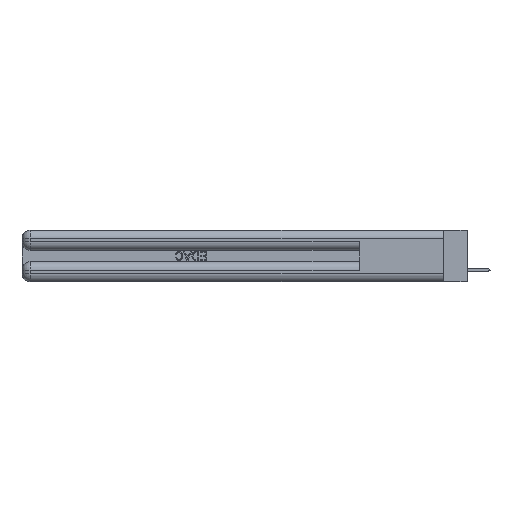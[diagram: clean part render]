
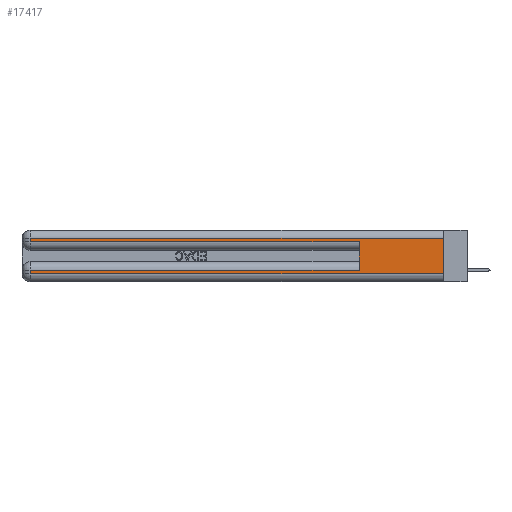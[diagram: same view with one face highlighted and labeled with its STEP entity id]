
A CAD part, left-side view. The second image highlights one B-rep face of the part: STEP entity #17417.
In plain terms, the highlighted planar face has unit normal (-1, 0, 0).
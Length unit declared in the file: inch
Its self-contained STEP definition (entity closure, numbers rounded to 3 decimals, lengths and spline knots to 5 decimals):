
#682 = VERTEX_POINT ( 'NONE', #5060 ) ;
#722 = DIRECTION ( 'NONE',  ( 0., -1., 0. ) ) ;
#943 = ORIENTED_EDGE ( 'NONE', *, *, #21924, .T. ) ;
#945 = DIRECTION ( 'NONE',  ( 0., 0., -1. ) ) ;
#1833 = DIRECTION ( 'NONE',  ( 0., 1., 0. ) ) ;
#3989 = ORIENTED_EDGE ( 'NONE', *, *, #22586, .T. ) ;
#4301 = DIRECTION ( 'NONE',  ( 0., 0., -1. ) ) ;
#4727 = CARTESIAN_POINT ( 'NONE',  ( 0., 0., 0.085 ) ) ;
#5060 = CARTESIAN_POINT ( 'NONE',  ( 0., 0.6, 0.085 ) ) ;
#5175 = CARTESIAN_POINT ( 'NONE',  ( 0., 2.94, 0.31 ) ) ;
#5986 = EDGE_LOOP ( 'NONE', ( #32829, #24049, #3989, #37953, #37852, #943, #38715, #15511 ) ) ;
#6036 = DIRECTION ( 'NONE',  ( 0., -1., 0. ) ) ;
#8787 = DIRECTION ( 'NONE',  ( 0., 0., 1. ) ) ;
#9273 = EDGE_CURVE ( 'NONE', #23100, #13949, #23487, .T. ) ;
#9518 = VERTEX_POINT ( 'NONE', #26101 ) ;
#10511 = EDGE_CURVE ( 'NONE', #9518, #33325, #34875, .T. ) ;
#10585 = DIRECTION ( 'NONE',  ( 1., 0., 0. ) ) ;
#11174 = EDGE_CURVE ( 'NONE', #23100, #39749, #25785, .T. ) ;
#11259 = CARTESIAN_POINT ( 'NONE',  ( 0., 0., 0.06 ) ) ;
#13336 = CARTESIAN_POINT ( 'NONE',  ( 0., 2.94, 0.37 ) ) ;
#13949 = VERTEX_POINT ( 'NONE', #11259 ) ;
#13953 = PLANE ( 'NONE',  #19264 ) ;
#14038 = DIRECTION ( 'NONE',  ( 0., 0., -1. ) ) ;
#14986 = VECTOR ( 'NONE', #8787, 39.37008 ) ;
#15511 = ORIENTED_EDGE ( 'NONE', *, *, #22435, .T. ) ;
#17315 = DIRECTION ( 'NONE',  ( 0., 0., -1. ) ) ;
#17417 = ADVANCED_FACE ( 'NONE', ( #29354 ), #13953, .F. ) ;
#17633 = CARTESIAN_POINT ( 'NONE',  ( 0., 2.94, 0.06 ) ) ;
#18669 = LINE ( 'NONE', #19816, #22580 ) ;
#19074 = VECTOR ( 'NONE', #14038, 39.37008 ) ;
#19264 = AXIS2_PLACEMENT_3D ( 'NONE', #36250, #10585, #17315 ) ;
#19464 = LINE ( 'NONE', #41075, #25459 ) ;
#19816 = CARTESIAN_POINT ( 'NONE',  ( 0., 0., 0.06 ) ) ;
#21317 = CARTESIAN_POINT ( 'NONE',  ( 0., 0.6, 0.145 ) ) ;
#21924 = EDGE_CURVE ( 'NONE', #682, #9518, #28683, .T. ) ;
#22400 = LINE ( 'NONE', #21317, #14986 ) ;
#22435 = EDGE_CURVE ( 'NONE', #33325, #13949, #18669, .T. ) ;
#22580 = VECTOR ( 'NONE', #722, 39.37008 ) ;
#22586 = EDGE_CURVE ( 'NONE', #39749, #40207, #29570, .T. ) ;
#23100 = VERTEX_POINT ( 'NONE', #27547 ) ;
#23487 = LINE ( 'NONE', #33095, #19074 ) ;
#23728 = CARTESIAN_POINT ( 'NONE',  ( 0., 2.94, 0.285 ) ) ;
#24049 = ORIENTED_EDGE ( 'NONE', *, *, #11174, .T. ) ;
#25459 = VECTOR ( 'NONE', #6036, 39.37008 ) ;
#25625 = VECTOR ( 'NONE', #1833, 39.37008 ) ;
#25785 = LINE ( 'NONE', #26768, #27336 ) ;
#26101 = CARTESIAN_POINT ( 'NONE',  ( 0., 2.94, 0.085 ) ) ;
#26768 = CARTESIAN_POINT ( 'NONE',  ( 0., 0., 0.31 ) ) ;
#27336 = VECTOR ( 'NONE', #40131, 39.37008 ) ;
#27547 = CARTESIAN_POINT ( 'NONE',  ( 0., 0., 0.31 ) ) ;
#28683 = LINE ( 'NONE', #4727, #25625 ) ;
#29103 = VECTOR ( 'NONE', #945, 39.37008 ) ;
#29332 = VERTEX_POINT ( 'NONE', #33403 ) ;
#29354 = FACE_OUTER_BOUND ( 'NONE', #5986, .T. ) ;
#29362 = EDGE_CURVE ( 'NONE', #682, #29332, #22400, .T. ) ;
#29570 = LINE ( 'NONE', #13336, #29103 ) ;
#32829 = ORIENTED_EDGE ( 'NONE', *, *, #9273, .F. ) ;
#33095 = CARTESIAN_POINT ( 'NONE',  ( 0., 0., 0.37 ) ) ;
#33325 = VERTEX_POINT ( 'NONE', #17633 ) ;
#33403 = CARTESIAN_POINT ( 'NONE',  ( 0., 0.6, 0.285 ) ) ;
#33562 = EDGE_CURVE ( 'NONE', #40207, #29332, #19464, .T. ) ;
#34875 = LINE ( 'NONE', #39158, #38369 ) ;
#36250 = CARTESIAN_POINT ( 'NONE',  ( 0., 0., 0.37 ) ) ;
#37852 = ORIENTED_EDGE ( 'NONE', *, *, #29362, .F. ) ;
#37953 = ORIENTED_EDGE ( 'NONE', *, *, #33562, .T. ) ;
#38369 = VECTOR ( 'NONE', #4301, 39.37008 ) ;
#38715 = ORIENTED_EDGE ( 'NONE', *, *, #10511, .T. ) ;
#39158 = CARTESIAN_POINT ( 'NONE',  ( 0., 2.94, 0.37 ) ) ;
#39749 = VERTEX_POINT ( 'NONE', #5175 ) ;
#40131 = DIRECTION ( 'NONE',  ( 0., 1., 0. ) ) ;
#40207 = VERTEX_POINT ( 'NONE', #23728 ) ;
#41075 = CARTESIAN_POINT ( 'NONE',  ( 0., 0., 0.285 ) ) ;
